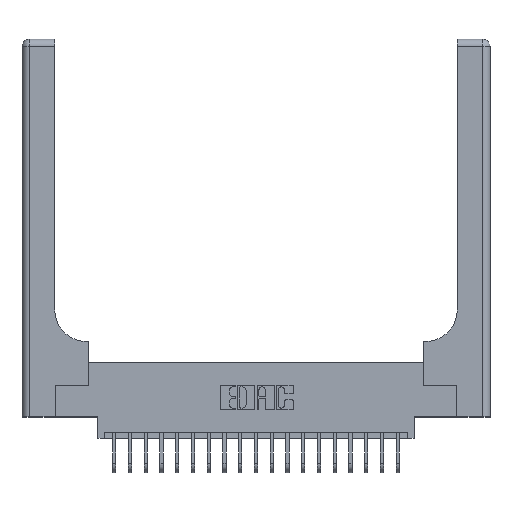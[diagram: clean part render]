
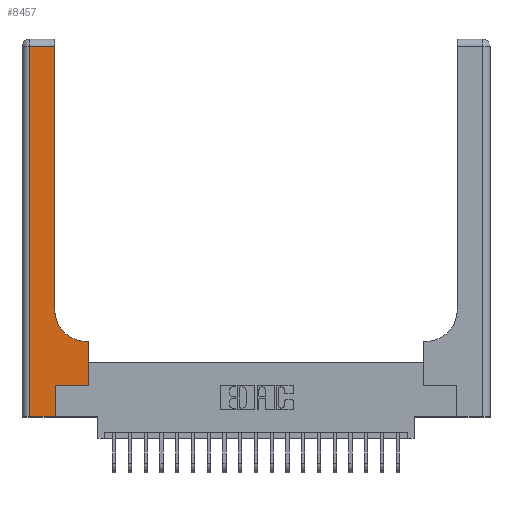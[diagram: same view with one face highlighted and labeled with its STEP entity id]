
A CAD part, top view. The second image highlights one B-rep face of the part: STEP entity #8457.
In plain terms, the highlighted planar face has unit normal (0, 0, 1).
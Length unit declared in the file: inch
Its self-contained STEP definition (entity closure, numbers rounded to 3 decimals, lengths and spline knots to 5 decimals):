
#62 = VERTEX_POINT ( 'NONE', #10987 ) ;
#559 = CARTESIAN_POINT ( 'NONE',  ( 0.265, 0.25, 0.37 ) ) ;
#701 = VERTEX_POINT ( 'NONE', #4137 ) ;
#812 = VECTOR ( 'NONE', #18660, 39.37008 ) ;
#1253 = LINE ( 'NONE', #18663, #13339 ) ;
#1684 = VERTEX_POINT ( 'NONE', #6604 ) ;
#2646 = CARTESIAN_POINT ( 'NONE',  ( 0.51, 0.6, 0.37 ) ) ;
#3014 = CARTESIAN_POINT ( 'NONE',  ( 0.26, 0.6, 0.37 ) ) ;
#3524 = DIRECTION ( 'NONE',  ( 0., 1., 0. ) ) ;
#3795 = VECTOR ( 'NONE', #3524, 39.37008 ) ;
#4137 = CARTESIAN_POINT ( 'NONE',  ( 0.528, 0.6, 0.37 ) ) ;
#4376 = CARTESIAN_POINT ( 'NONE',  ( 0., 0., 0.37 ) ) ;
#4455 = ORIENTED_EDGE ( 'NONE', *, *, #7906, .T. ) ;
#4527 = CARTESIAN_POINT ( 'NONE',  ( 0.26, 3., 0.37 ) ) ;
#5114 = CARTESIAN_POINT ( 'NONE',  ( 0.51, 0.85, 0.37 ) ) ;
#5304 = VECTOR ( 'NONE', #13878, 39.37008 ) ;
#5901 = ORIENTED_EDGE ( 'NONE', *, *, #18369, .T. ) ;
#6007 = VECTOR ( 'NONE', #16852, 39.37008 ) ;
#6255 = VERTEX_POINT ( 'NONE', #14787 ) ;
#6267 = VERTEX_POINT ( 'NONE', #19448 ) ;
#6393 = ORIENTED_EDGE ( 'NONE', *, *, #9346, .T. ) ;
#6604 = CARTESIAN_POINT ( 'NONE',  ( 0.528, 0.25, 0.37 ) ) ;
#6668 = DIRECTION ( 'NONE',  ( 1., 0., 0. ) ) ;
#6745 = EDGE_CURVE ( 'NONE', #701, #11674, #17058, .T. ) ;
#7062 = VERTEX_POINT ( 'NONE', #11717 ) ;
#7465 = FACE_OUTER_BOUND ( 'NONE', #10507, .T. ) ;
#7906 = EDGE_CURVE ( 'NONE', #6267, #62, #17255, .T. ) ;
#7912 = CIRCLE ( 'NONE', #20087, 0.25 ) ;
#8175 = CARTESIAN_POINT ( 'NONE',  ( 0., 2.94, 0.37 ) ) ;
#8186 = CARTESIAN_POINT ( 'NONE',  ( 0.528, 0.25, 0.37 ) ) ;
#8457 = ADVANCED_FACE ( 'NONE', ( #7465 ), #15214, .F. ) ;
#8574 = EDGE_CURVE ( 'NONE', #6255, #7062, #1253, .T. ) ;
#8598 = ORIENTED_EDGE ( 'NONE', *, *, #12510, .T. ) ;
#8999 = DIRECTION ( 'NONE',  ( -1., 0., 0. ) ) ;
#9095 = ORIENTED_EDGE ( 'NONE', *, *, #17983, .T. ) ;
#9346 = EDGE_CURVE ( 'NONE', #11674, #6267, #7912, .T. ) ;
#9733 = DIRECTION ( 'NONE',  ( -1., 0., 0. ) ) ;
#10063 = ORIENTED_EDGE ( 'NONE', *, *, #6745, .T. ) ;
#10507 = EDGE_LOOP ( 'NONE', ( #4455, #8598, #12762, #9095, #17395, #17870, #5901, #10063, #6393 ) ) ;
#10554 = EDGE_CURVE ( 'NONE', #7062, #1684, #14952, .T. ) ;
#10723 = VECTOR ( 'NONE', #9733, 39.37008 ) ;
#10987 = CARTESIAN_POINT ( 'NONE',  ( 0.26, 2.94, 0.37 ) ) ;
#11314 = VECTOR ( 'NONE', #14680, 39.37008 ) ;
#11462 = EDGE_CURVE ( 'NONE', #17007, #13794, #19988, .T. ) ;
#11674 = VERTEX_POINT ( 'NONE', #2646 ) ;
#11717 = CARTESIAN_POINT ( 'NONE',  ( 0.265, 0.25, 0.37 ) ) ;
#11747 = VECTOR ( 'NONE', #16068, 39.37008 ) ;
#12510 = EDGE_CURVE ( 'NONE', #62, #17007, #14866, .T. ) ;
#12622 = LINE ( 'NONE', #8186, #3795 ) ;
#12762 = ORIENTED_EDGE ( 'NONE', *, *, #11462, .T. ) ;
#13339 = VECTOR ( 'NONE', #16976, 39.37008 ) ;
#13794 = VERTEX_POINT ( 'NONE', #17932 ) ;
#13878 = DIRECTION ( 'NONE',  ( 0., 1., 0. ) ) ;
#14680 = DIRECTION ( 'NONE',  ( 1., 0., 0. ) ) ;
#14787 = CARTESIAN_POINT ( 'NONE',  ( 0.265, 0., 0.37 ) ) ;
#14866 = LINE ( 'NONE', #8175, #10723 ) ;
#14952 = LINE ( 'NONE', #559, #11314 ) ;
#15214 = PLANE ( 'NONE',  #17773 ) ;
#16022 = DIRECTION ( 'NONE',  ( 0., 0., -1. ) ) ;
#16068 = DIRECTION ( 'NONE',  ( 0., -1., 0. ) ) ;
#16769 = CARTESIAN_POINT ( 'NONE',  ( 0., 3., 0.37 ) ) ;
#16852 = DIRECTION ( 'NONE',  ( 1., 0., 0. ) ) ;
#16976 = DIRECTION ( 'NONE',  ( 0., 1., 0. ) ) ;
#17007 = VERTEX_POINT ( 'NONE', #19720 ) ;
#17058 = LINE ( 'NONE', #3014, #812 ) ;
#17255 = LINE ( 'NONE', #4527, #5304 ) ;
#17395 = ORIENTED_EDGE ( 'NONE', *, *, #8574, .T. ) ;
#17568 = CARTESIAN_POINT ( 'NONE',  ( 0.06, 3., 0.37 ) ) ;
#17773 = AXIS2_PLACEMENT_3D ( 'NONE', #16769, #18340, #8999 ) ;
#17870 = ORIENTED_EDGE ( 'NONE', *, *, #10554, .T. ) ;
#17932 = CARTESIAN_POINT ( 'NONE',  ( 0.06, 0., 0.37 ) ) ;
#17983 = EDGE_CURVE ( 'NONE', #13794, #6255, #19410, .T. ) ;
#18340 = DIRECTION ( 'NONE',  ( 0., 0., -1. ) ) ;
#18369 = EDGE_CURVE ( 'NONE', #1684, #701, #12622, .T. ) ;
#18660 = DIRECTION ( 'NONE',  ( -1., 0., 0. ) ) ;
#18663 = CARTESIAN_POINT ( 'NONE',  ( 0.265, 0., 0.37 ) ) ;
#19410 = LINE ( 'NONE', #4376, #6007 ) ;
#19448 = CARTESIAN_POINT ( 'NONE',  ( 0.26, 0.85, 0.37 ) ) ;
#19720 = CARTESIAN_POINT ( 'NONE',  ( 0.06, 2.94, 0.37 ) ) ;
#19988 = LINE ( 'NONE', #17568, #11747 ) ;
#20087 = AXIS2_PLACEMENT_3D ( 'NONE', #5114, #16022, #6668 ) ;
